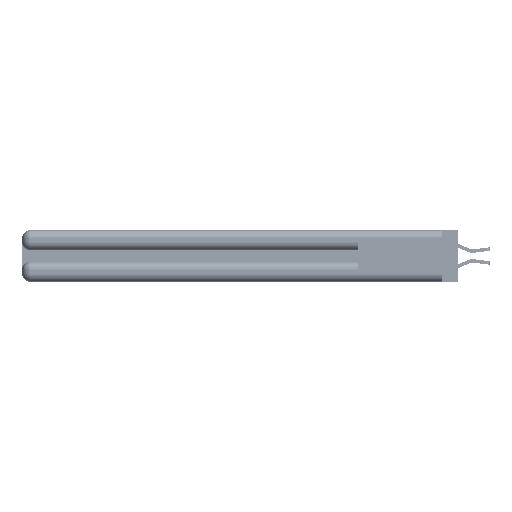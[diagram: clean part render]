
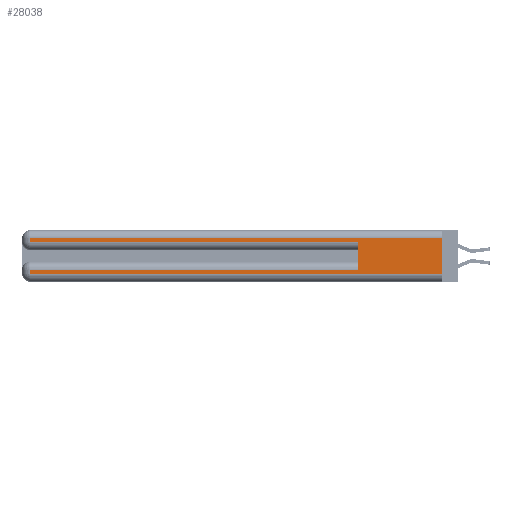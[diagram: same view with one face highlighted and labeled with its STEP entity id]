
A CAD part, left-side view. The second image highlights one B-rep face of the part: STEP entity #28038.
In plain terms, the highlighted planar face has unit normal (-1, 0, 0).
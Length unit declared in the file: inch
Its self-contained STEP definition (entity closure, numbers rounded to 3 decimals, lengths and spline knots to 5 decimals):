
#958 = LINE ( 'NONE', #5585, #10785 ) ;
#2863 = ORIENTED_EDGE ( 'NONE', *, *, #22122, .F. ) ;
#2880 = AXIS2_PLACEMENT_3D ( 'NONE', #3149, #35003, #38931 ) ;
#3149 = CARTESIAN_POINT ( 'NONE',  ( 0., 0., 0.37 ) ) ;
#3239 = ORIENTED_EDGE ( 'NONE', *, *, #12367, .F. ) ;
#3593 = CARTESIAN_POINT ( 'NONE',  ( 0., 0., 0.06 ) ) ;
#3744 = LINE ( 'NONE', #6756, #44406 ) ;
#4766 = CARTESIAN_POINT ( 'NONE',  ( 0., 2.94, 0.37 ) ) ;
#5214 = DIRECTION ( 'NONE',  ( 0., 0., 1. ) ) ;
#5585 = CARTESIAN_POINT ( 'NONE',  ( 0., 0., 0.31 ) ) ;
#6420 = CARTESIAN_POINT ( 'NONE',  ( 0., 0., 0.285 ) ) ;
#6711 = VECTOR ( 'NONE', #27555, 39.37008 ) ;
#6756 = CARTESIAN_POINT ( 'NONE',  ( 0., 2.94, 0.37 ) ) ;
#7118 = VECTOR ( 'NONE', #5214, 39.37008 ) ;
#7140 = PLANE ( 'NONE',  #2880 ) ;
#9962 = LINE ( 'NONE', #17004, #33361 ) ;
#10785 = VECTOR ( 'NONE', #40997, 39.37008 ) ;
#11229 = CARTESIAN_POINT ( 'NONE',  ( 0., 0.6, 0.085 ) ) ;
#11257 = CARTESIAN_POINT ( 'NONE',  ( 0., 0., 0.085 ) ) ;
#11530 = ORIENTED_EDGE ( 'NONE', *, *, #19257, .T. ) ;
#12154 = VERTEX_POINT ( 'NONE', #14954 ) ;
#12367 = EDGE_CURVE ( 'NONE', #46283, #22165, #9962, .T. ) ;
#12610 = LINE ( 'NONE', #6420, #50709 ) ;
#12762 = CARTESIAN_POINT ( 'NONE',  ( 0., 0.6, 0.285 ) ) ;
#13310 = LINE ( 'NONE', #48541, #7118 ) ;
#14669 = VERTEX_POINT ( 'NONE', #41591 ) ;
#14855 = DIRECTION ( 'NONE',  ( 0., -1., 0. ) ) ;
#14954 = CARTESIAN_POINT ( 'NONE',  ( 0., 2.94, 0.285 ) ) ;
#15463 = EDGE_CURVE ( 'NONE', #48148, #14669, #43511, .T. ) ;
#16306 = DIRECTION ( 'NONE',  ( 0., 0., -1. ) ) ;
#16461 = CARTESIAN_POINT ( 'NONE',  ( 0., 2.94, 0.31 ) ) ;
#17004 = CARTESIAN_POINT ( 'NONE',  ( 0., 0., 0.37 ) ) ;
#17699 = ORIENTED_EDGE ( 'NONE', *, *, #15463, .T. ) ;
#18281 = DIRECTION ( 'NONE',  ( 0., 0., -1. ) ) ;
#19257 = EDGE_CURVE ( 'NONE', #14669, #30943, #3744, .T. ) ;
#19930 = ORIENTED_EDGE ( 'NONE', *, *, #42353, .T. ) ;
#20067 = DIRECTION ( 'NONE',  ( 0., 0., -1. ) ) ;
#21689 = VECTOR ( 'NONE', #16306, 39.37008 ) ;
#22122 = EDGE_CURVE ( 'NONE', #48148, #49727, #13310, .T. ) ;
#22165 = VERTEX_POINT ( 'NONE', #33584 ) ;
#25083 = VECTOR ( 'NONE', #38748, 39.37008 ) ;
#26386 = CARTESIAN_POINT ( 'NONE',  ( 0., 0., 0.31 ) ) ;
#27342 = ORIENTED_EDGE ( 'NONE', *, *, #31670, .T. ) ;
#27555 = DIRECTION ( 'NONE',  ( 0., -1., 0. ) ) ;
#28038 = ADVANCED_FACE ( 'NONE', ( #28080 ), #7140, .F. ) ;
#28080 = FACE_OUTER_BOUND ( 'NONE', #44050, .T. ) ;
#30943 = VERTEX_POINT ( 'NONE', #31011 ) ;
#31011 = CARTESIAN_POINT ( 'NONE',  ( 0., 2.94, 0.06 ) ) ;
#31670 = EDGE_CURVE ( 'NONE', #30943, #22165, #33197, .T. ) ;
#33197 = LINE ( 'NONE', #3593, #6711 ) ;
#33361 = VECTOR ( 'NONE', #20067, 39.37008 ) ;
#33524 = ORIENTED_EDGE ( 'NONE', *, *, #40739, .T. ) ;
#33584 = CARTESIAN_POINT ( 'NONE',  ( 0., 0., 0.06 ) ) ;
#35003 = DIRECTION ( 'NONE',  ( 1., 0., 0. ) ) ;
#36497 = ORIENTED_EDGE ( 'NONE', *, *, #47206, .T. ) ;
#38748 = DIRECTION ( 'NONE',  ( 0., 1., 0. ) ) ;
#38931 = DIRECTION ( 'NONE',  ( 0., 0., -1. ) ) ;
#40739 = EDGE_CURVE ( 'NONE', #46283, #48455, #958, .T. ) ;
#40997 = DIRECTION ( 'NONE',  ( 0., 1., 0. ) ) ;
#41591 = CARTESIAN_POINT ( 'NONE',  ( 0., 2.94, 0.085 ) ) ;
#42353 = EDGE_CURVE ( 'NONE', #12154, #49727, #12610, .T. ) ;
#43511 = LINE ( 'NONE', #11257, #25083 ) ;
#44050 = EDGE_LOOP ( 'NONE', ( #3239, #33524, #36497, #19930, #2863, #17699, #11530, #27342 ) ) ;
#44406 = VECTOR ( 'NONE', #18281, 39.37008 ) ;
#45096 = LINE ( 'NONE', #4766, #21689 ) ;
#46283 = VERTEX_POINT ( 'NONE', #26386 ) ;
#47206 = EDGE_CURVE ( 'NONE', #48455, #12154, #45096, .T. ) ;
#48148 = VERTEX_POINT ( 'NONE', #11229 ) ;
#48455 = VERTEX_POINT ( 'NONE', #16461 ) ;
#48541 = CARTESIAN_POINT ( 'NONE',  ( 0., 0.6, 0.145 ) ) ;
#49727 = VERTEX_POINT ( 'NONE', #12762 ) ;
#50709 = VECTOR ( 'NONE', #14855, 39.37008 ) ;
